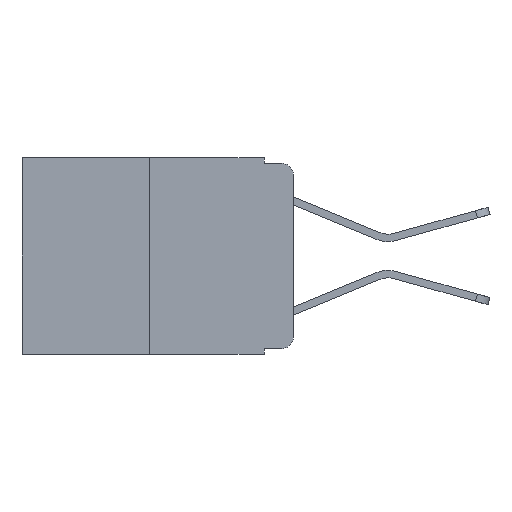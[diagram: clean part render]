
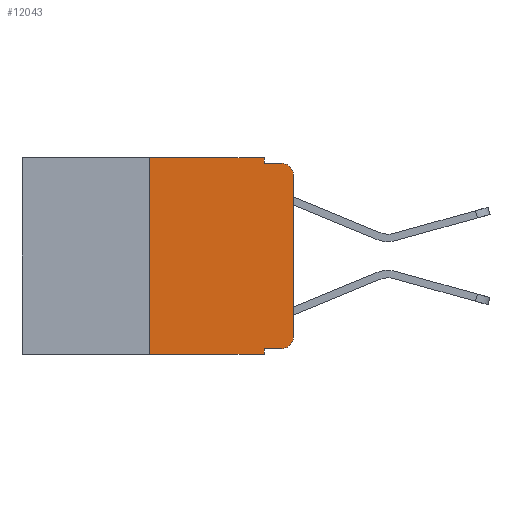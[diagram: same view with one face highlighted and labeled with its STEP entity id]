
A CAD part, left-side view. The second image highlights one B-rep face of the part: STEP entity #12043.
In plain terms, the highlighted planar face has unit normal (-1, 0, 0).
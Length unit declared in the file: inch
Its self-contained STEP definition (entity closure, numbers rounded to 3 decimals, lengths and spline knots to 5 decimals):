
#14 = EDGE_CURVE ( 'NONE', #7487, #45, #6701, .T. ) ;
#45 = VERTEX_POINT ( 'NONE', #206 ) ;
#138 = CARTESIAN_POINT ( 'NONE',  ( 0., 0.051, -0.333 ) ) ;
#206 = CARTESIAN_POINT ( 'NONE',  ( 0., 0.051, -0.343 ) ) ;
#249 = VERTEX_POINT ( 'NONE', #7511 ) ;
#277 = ORIENTED_EDGE ( 'NONE', *, *, #6962, .T. ) ;
#301 = ORIENTED_EDGE ( 'NONE', *, *, #1591, .F. ) ;
#431 = ORIENTED_EDGE ( 'NONE', *, *, #11157, .T. ) ;
#663 = VECTOR ( 'NONE', #5160, 39.37008 ) ;
#677 = DIRECTION ( 'NONE',  ( 1., 0., 0. ) ) ;
#751 = VERTEX_POINT ( 'NONE', #4679 ) ;
#797 = ORIENTED_EDGE ( 'NONE', *, *, #8059, .F. ) ;
#893 = DIRECTION ( 'NONE',  ( 0., 0., -1. ) ) ;
#1000 = CARTESIAN_POINT ( 'NONE',  ( 0., 0.02, -0.333 ) ) ;
#1142 = DIRECTION ( 'NONE',  ( 0., -1., 0. ) ) ;
#1513 = LINE ( 'NONE', #5941, #3993 ) ;
#1591 = EDGE_CURVE ( 'NONE', #7401, #6259, #9255, .T. ) ;
#1755 = LINE ( 'NONE', #10779, #6770 ) ;
#2242 = VERTEX_POINT ( 'NONE', #6113 ) ;
#2355 = DIRECTION ( 'NONE',  ( 0., 0., 1. ) ) ;
#2370 = ORIENTED_EDGE ( 'NONE', *, *, #11732, .T. ) ;
#2757 = FACE_OUTER_BOUND ( 'NONE', #4926, .T. ) ;
#2855 = DIRECTION ( 'NONE',  ( -1., 0., 0. ) ) ;
#2912 = VERTEX_POINT ( 'NONE', #10309 ) ;
#3107 = ORIENTED_EDGE ( 'NONE', *, *, #6338, .T. ) ;
#3552 = DIRECTION ( 'NONE',  ( 0., -1., 0. ) ) ;
#3614 = DIRECTION ( 'NONE',  ( 0., -1., 0. ) ) ;
#3728 = EDGE_CURVE ( 'NONE', #4323, #751, #10760, .T. ) ;
#3893 = CARTESIAN_POINT ( 'NONE',  ( 0., 0.473, 0. ) ) ;
#3993 = VECTOR ( 'NONE', #11987, 39.37008 ) ;
#4257 = CIRCLE ( 'NONE', #10669, 0.02 ) ;
#4323 = VERTEX_POINT ( 'NONE', #5490 ) ;
#4679 = CARTESIAN_POINT ( 'NONE',  ( 0., 0.051, -0.01 ) ) ;
#4926 = EDGE_LOOP ( 'NONE', ( #277, #3107, #8564, #8902, #797, #301, #11601, #5967, #2370, #431 ) ) ;
#4942 = LINE ( 'NONE', #9941, #11673 ) ;
#5062 = EDGE_CURVE ( 'NONE', #751, #2242, #1513, .T. ) ;
#5160 = DIRECTION ( 'NONE',  ( 0., 0., -1. ) ) ;
#5170 = CARTESIAN_POINT ( 'NONE',  ( 0., 0.051, 0. ) ) ;
#5490 = CARTESIAN_POINT ( 'NONE',  ( 0., 0.051, 0. ) ) ;
#5583 = AXIS2_PLACEMENT_3D ( 'NONE', #8499, #2855, #9354 ) ;
#5690 = CARTESIAN_POINT ( 'NONE',  ( 0., 0., 0. ) ) ;
#5748 = LINE ( 'NONE', #8927, #10136 ) ;
#5822 = VERTEX_POINT ( 'NONE', #1000 ) ;
#5941 = CARTESIAN_POINT ( 'NONE',  ( 0., 0.051, -0.01 ) ) ;
#5967 = ORIENTED_EDGE ( 'NONE', *, *, #14, .F. ) ;
#6096 = VECTOR ( 'NONE', #8313, 39.37008 ) ;
#6113 = CARTESIAN_POINT ( 'NONE',  ( 0., 0.02, -0.01 ) ) ;
#6259 = VERTEX_POINT ( 'NONE', #9346 ) ;
#6338 = EDGE_CURVE ( 'NONE', #249, #2242, #4257, .T. ) ;
#6428 = CARTESIAN_POINT ( 'NONE',  ( 0., 0.25, 0. ) ) ;
#6701 = LINE ( 'NONE', #10831, #6096 ) ;
#6770 = VECTOR ( 'NONE', #3614, 39.37008 ) ;
#6818 = PLANE ( 'NONE',  #7949 ) ;
#6895 = CIRCLE ( 'NONE', #5583, 0.02 ) ;
#6962 = EDGE_CURVE ( 'NONE', #2912, #249, #9120, .T. ) ;
#6972 = DIRECTION ( 'NONE',  ( -1., 0., 0. ) ) ;
#7401 = VERTEX_POINT ( 'NONE', #8061 ) ;
#7487 = VERTEX_POINT ( 'NONE', #138 ) ;
#7511 = CARTESIAN_POINT ( 'NONE',  ( 0., 0., -0.03 ) ) ;
#7691 = DIRECTION ( 'NONE',  ( 0., 0., -1. ) ) ;
#7949 = AXIS2_PLACEMENT_3D ( 'NONE', #3893, #677, #7691 ) ;
#8059 = EDGE_CURVE ( 'NONE', #6259, #4323, #5748, .T. ) ;
#8061 = CARTESIAN_POINT ( 'NONE',  ( 0., 0.25, -0.343 ) ) ;
#8313 = DIRECTION ( 'NONE',  ( 0., 0., -1. ) ) ;
#8499 = CARTESIAN_POINT ( 'NONE',  ( 0., 0.02, -0.313 ) ) ;
#8564 = ORIENTED_EDGE ( 'NONE', *, *, #5062, .F. ) ;
#8855 = VECTOR ( 'NONE', #10105, 39.37008 ) ;
#8902 = ORIENTED_EDGE ( 'NONE', *, *, #3728, .F. ) ;
#8927 = CARTESIAN_POINT ( 'NONE',  ( 0., 0.473, 0. ) ) ;
#9120 = LINE ( 'NONE', #5690, #8855 ) ;
#9255 = LINE ( 'NONE', #6428, #9519 ) ;
#9346 = CARTESIAN_POINT ( 'NONE',  ( 0., 0.25, 0. ) ) ;
#9354 = DIRECTION ( 'NONE',  ( 0., 0., -1. ) ) ;
#9519 = VECTOR ( 'NONE', #2355, 39.37008 ) ;
#9941 = CARTESIAN_POINT ( 'NONE',  ( 0., 0.051, -0.333 ) ) ;
#10105 = DIRECTION ( 'NONE',  ( 0., 0., 1. ) ) ;
#10136 = VECTOR ( 'NONE', #1142, 39.37008 ) ;
#10185 = EDGE_CURVE ( 'NONE', #7401, #45, #1755, .T. ) ;
#10309 = CARTESIAN_POINT ( 'NONE',  ( 0., 0., -0.313 ) ) ;
#10669 = AXIS2_PLACEMENT_3D ( 'NONE', #12074, #6972, #893 ) ;
#10760 = LINE ( 'NONE', #5170, #663 ) ;
#10779 = CARTESIAN_POINT ( 'NONE',  ( 0., 0.473, -0.343 ) ) ;
#10831 = CARTESIAN_POINT ( 'NONE',  ( 0., 0.051, 0. ) ) ;
#11157 = EDGE_CURVE ( 'NONE', #5822, #2912, #6895, .T. ) ;
#11601 = ORIENTED_EDGE ( 'NONE', *, *, #10185, .T. ) ;
#11673 = VECTOR ( 'NONE', #3552, 39.37008 ) ;
#11732 = EDGE_CURVE ( 'NONE', #7487, #5822, #4942, .T. ) ;
#11987 = DIRECTION ( 'NONE',  ( 0., -1., 0. ) ) ;
#12043 = ADVANCED_FACE ( 'NONE', ( #2757 ), #6818, .F. ) ;
#12074 = CARTESIAN_POINT ( 'NONE',  ( 0., 0.02, -0.03 ) ) ;
